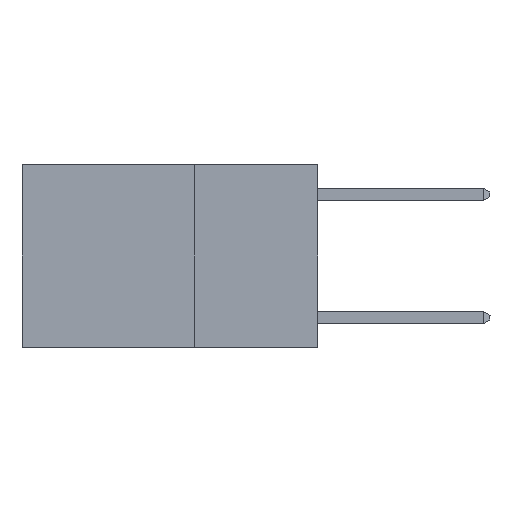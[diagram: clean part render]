
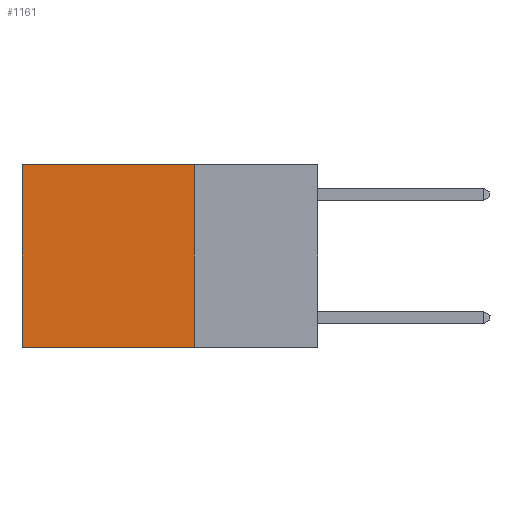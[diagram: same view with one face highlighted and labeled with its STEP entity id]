
A CAD part, left-side view. The second image highlights one B-rep face of the part: STEP entity #1161.
In plain terms, the highlighted planar face has unit normal (-1, 0, 0).
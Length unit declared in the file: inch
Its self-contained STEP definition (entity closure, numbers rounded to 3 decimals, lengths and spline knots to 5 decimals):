
#597 = LINE ( 'NONE', #5204, #13341 ) ;
#677 = ORIENTED_EDGE ( 'NONE', *, *, #3701, .F. ) ;
#1161 = ADVANCED_FACE ( 'NONE', ( #7007 ), #7462, .F. ) ;
#2145 = ORIENTED_EDGE ( 'NONE', *, *, #4604, .T. ) ;
#2651 = VECTOR ( 'NONE', #2684, 39.37008 ) ;
#2684 = DIRECTION ( 'NONE',  ( 0., 1., 0. ) ) ;
#2936 = VERTEX_POINT ( 'NONE', #16593 ) ;
#3462 = VECTOR ( 'NONE', #8989, 39.37008 ) ;
#3478 = VERTEX_POINT ( 'NONE', #19493 ) ;
#3701 = EDGE_CURVE ( 'NONE', #14470, #10491, #18673, .T. ) ;
#4263 = CARTESIAN_POINT ( 'NONE',  ( 0.2625, 0.25, 0. ) ) ;
#4287 = EDGE_CURVE ( 'NONE', #3478, #10491, #597, .T. ) ;
#4604 = EDGE_CURVE ( 'NONE', #2936, #3478, #11547, .T. ) ;
#5204 = CARTESIAN_POINT ( 'NONE',  ( 0.2625, 0.6, 0. ) ) ;
#5919 = DIRECTION ( 'NONE',  ( 0., 0., -1. ) ) ;
#7007 = FACE_OUTER_BOUND ( 'NONE', #7428, .T. ) ;
#7247 = CARTESIAN_POINT ( 'NONE',  ( 0.2625, 0.25, 0. ) ) ;
#7428 = EDGE_LOOP ( 'NONE', ( #8647, #677, #20641, #2145 ) ) ;
#7462 = PLANE ( 'NONE',  #8401 ) ;
#8401 = AXIS2_PLACEMENT_3D ( 'NONE', #4263, #15803, #5919 ) ;
#8647 = ORIENTED_EDGE ( 'NONE', *, *, #4287, .T. ) ;
#8989 = DIRECTION ( 'NONE',  ( 0., 0., -1. ) ) ;
#9033 = CARTESIAN_POINT ( 'NONE',  ( 0.2625, 0.25, -0.37 ) ) ;
#9210 = CARTESIAN_POINT ( 'NONE',  ( 0.2625, 0.6, -0.37 ) ) ;
#10226 = DIRECTION ( 'NONE',  ( 0., 0., -1. ) ) ;
#10491 = VERTEX_POINT ( 'NONE', #9210 ) ;
#11547 = LINE ( 'NONE', #19117, #2651 ) ;
#11808 = LINE ( 'NONE', #7247, #3462 ) ;
#13341 = VECTOR ( 'NONE', #10226, 39.37008 ) ;
#14398 = VECTOR ( 'NONE', #19963, 39.37008 ) ;
#14470 = VERTEX_POINT ( 'NONE', #9033 ) ;
#15803 = DIRECTION ( 'NONE',  ( 1., 0., 0. ) ) ;
#16593 = CARTESIAN_POINT ( 'NONE',  ( 0.2625, 0.25, 0. ) ) ;
#17057 = EDGE_CURVE ( 'NONE', #2936, #14470, #11808, .T. ) ;
#18363 = CARTESIAN_POINT ( 'NONE',  ( 0.2625, 0.25, -0.37 ) ) ;
#18673 = LINE ( 'NONE', #18363, #14398 ) ;
#19117 = CARTESIAN_POINT ( 'NONE',  ( 0.2625, 0.25, 0. ) ) ;
#19493 = CARTESIAN_POINT ( 'NONE',  ( 0.2625, 0.6, 0. ) ) ;
#19963 = DIRECTION ( 'NONE',  ( 0., 1., 0. ) ) ;
#20641 = ORIENTED_EDGE ( 'NONE', *, *, #17057, .F. ) ;
